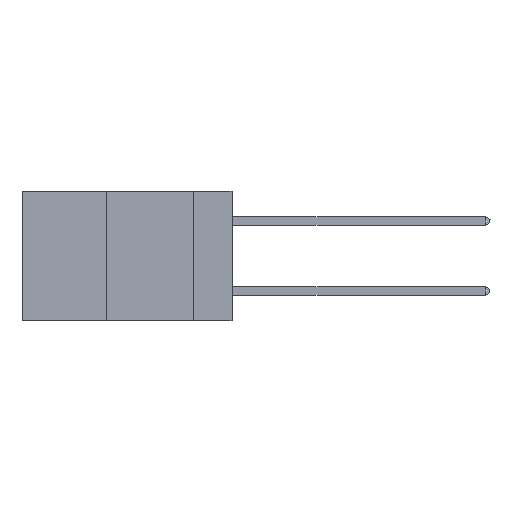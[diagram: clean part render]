
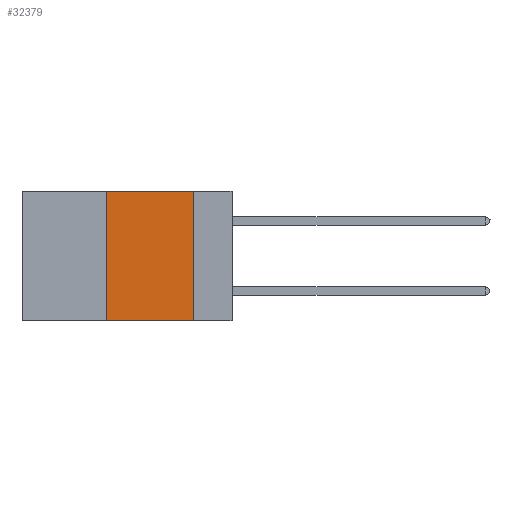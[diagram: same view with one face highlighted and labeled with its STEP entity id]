
A CAD part, left-side view. The second image highlights one B-rep face of the part: STEP entity #32379.
In plain terms, the highlighted planar face has unit normal (-1, 0, 0).
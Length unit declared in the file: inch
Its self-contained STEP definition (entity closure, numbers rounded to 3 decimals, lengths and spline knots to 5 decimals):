
#1557 = FACE_OUTER_BOUND ( 'NONE', #5653, .T. ) ;
#3397 = CARTESIAN_POINT ( 'NONE',  ( 0., 0.6, 0. ) ) ;
#4231 = AXIS2_PLACEMENT_3D ( 'NONE', #35167, #17830, #7589 ) ;
#5653 = EDGE_LOOP ( 'NONE', ( #31035, #23057, #26455, #19353 ) ) ;
#6984 = DIRECTION ( 'NONE',  ( 0., 0., -1. ) ) ;
#7424 = CARTESIAN_POINT ( 'NONE',  ( 0., 0.11, 0. ) ) ;
#7589 = DIRECTION ( 'NONE',  ( 0., 0., -1. ) ) ;
#8971 = CARTESIAN_POINT ( 'NONE',  ( 0., 0.36, 0. ) ) ;
#9445 = CARTESIAN_POINT ( 'NONE',  ( 0., 0.11, 0. ) ) ;
#13439 = DIRECTION ( 'NONE',  ( 0., -1., 0. ) ) ;
#15156 = PLANE ( 'NONE',  #4231 ) ;
#15426 = CARTESIAN_POINT ( 'NONE',  ( 0., 0.36, 0. ) ) ;
#16081 = LINE ( 'NONE', #15426, #36756 ) ;
#16492 = DIRECTION ( 'NONE',  ( 0., -1., 0. ) ) ;
#17830 = DIRECTION ( 'NONE',  ( 1., 0., 0. ) ) ;
#19353 = ORIENTED_EDGE ( 'NONE', *, *, #24023, .T. ) ;
#20320 = LINE ( 'NONE', #3397, #40000 ) ;
#22424 = VERTEX_POINT ( 'NONE', #8971 ) ;
#23057 = ORIENTED_EDGE ( 'NONE', *, *, #41069, .F. ) ;
#23817 = CARTESIAN_POINT ( 'NONE',  ( 0., 0.6, -0.37 ) ) ;
#23842 = VECTOR ( 'NONE', #6984, 39.37008 ) ;
#24023 = EDGE_CURVE ( 'NONE', #42652, #38945, #34053, .T. ) ;
#26455 = ORIENTED_EDGE ( 'NONE', *, *, #30641, .F. ) ;
#26505 = CARTESIAN_POINT ( 'NONE',  ( 0., 0.36, -0.37 ) ) ;
#29003 = EDGE_CURVE ( 'NONE', #30560, #38945, #37234, .T. ) ;
#30560 = VERTEX_POINT ( 'NONE', #7424 ) ;
#30641 = EDGE_CURVE ( 'NONE', #42652, #22424, #16081, .T. ) ;
#31035 = ORIENTED_EDGE ( 'NONE', *, *, #29003, .F. ) ;
#32094 = DIRECTION ( 'NONE',  ( 0., 0., 1. ) ) ;
#32379 = ADVANCED_FACE ( 'NONE', ( #1557 ), #15156, .F. ) ;
#34053 = LINE ( 'NONE', #23817, #37221 ) ;
#35167 = CARTESIAN_POINT ( 'NONE',  ( 0., 0.6, 0. ) ) ;
#36756 = VECTOR ( 'NONE', #32094, 39.37008 ) ;
#37221 = VECTOR ( 'NONE', #16492, 39.37008 ) ;
#37234 = LINE ( 'NONE', #9445, #23842 ) ;
#38945 = VERTEX_POINT ( 'NONE', #43746 ) ;
#40000 = VECTOR ( 'NONE', #13439, 39.37008 ) ;
#41069 = EDGE_CURVE ( 'NONE', #22424, #30560, #20320, .T. ) ;
#42652 = VERTEX_POINT ( 'NONE', #26505 ) ;
#43746 = CARTESIAN_POINT ( 'NONE',  ( 0., 0.11, -0.37 ) ) ;
